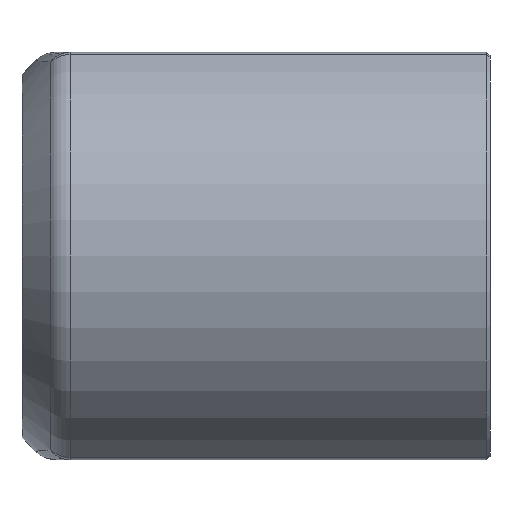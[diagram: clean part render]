
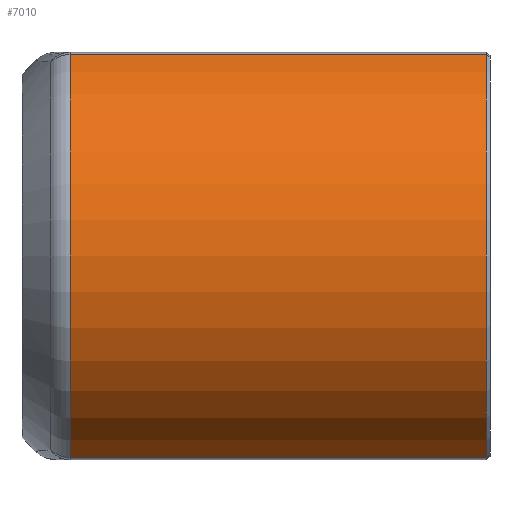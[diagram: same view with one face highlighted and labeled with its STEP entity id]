
A CAD part, front view. The second image highlights one B-rep face of the part: STEP entity #7010.
In plain terms, the highlighted cylindrical face has radius 23.709 mm (diameter 47.418 mm), a partial arc.
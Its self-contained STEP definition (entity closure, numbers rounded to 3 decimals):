
#155 = AXIS2_PLACEMENT_3D ( 'NONE', #1869, #4027, #1839 ) ;
#312 = CARTESIAN_POINT ( 'NONE',  ( -276.425, 16.131, -22.064 ) ) ;
#681 = DIRECTION ( 'NONE',  ( -1., 0., 0. ) ) ;
#938 = VERTEX_POINT ( 'NONE', #7049 ) ;
#957 = FACE_OUTER_BOUND ( 'NONE', #5071, .T. ) ;
#1297 = ORIENTED_EDGE ( 'NONE', *, *, #4584, .F. ) ;
#1752 = VECTOR ( 'NONE', #681, 1000. ) ;
#1839 = DIRECTION ( 'NONE',  ( 0., 0., 1. ) ) ;
#1869 = CARTESIAN_POINT ( 'NONE',  ( -231.416, 25.482, -0.277 ) ) ;
#1878 = LINE ( 'NONE', #5537, #8579 ) ;
#3190 = CARTESIAN_POINT ( 'NONE',  ( -231.416, 16.131, 21.51 ) ) ;
#3499 = CARTESIAN_POINT ( 'NONE',  ( -246.285, 25.482, -0.277 ) ) ;
#3546 = DIRECTION ( 'NONE',  ( -1., 0., 0. ) ) ;
#4027 = DIRECTION ( 'NONE',  ( 1., 0., 0. ) ) ;
#4071 = DIRECTION ( 'NONE',  ( -1., 0., 0. ) ) ;
#4508 = ORIENTED_EDGE ( 'NONE', *, *, #6011, .T. ) ;
#4584 = EDGE_CURVE ( 'NONE', #4763, #6753, #8475, .T. ) ;
#4763 = VERTEX_POINT ( 'NONE', #3190 ) ;
#5071 = EDGE_LOOP ( 'NONE', ( #5627, #5178, #1297, #4508 ) ) ;
#5132 = EDGE_CURVE ( 'NONE', #6753, #5558, #1878, .T. ) ;
#5178 = ORIENTED_EDGE ( 'NONE', *, *, #5132, .F. ) ;
#5341 = CYLINDRICAL_SURFACE ( 'NONE', #7238, 23.709 ) ;
#5537 = CARTESIAN_POINT ( 'NONE',  ( -246.285, 16.131, -22.064 ) ) ;
#5558 = VERTEX_POINT ( 'NONE', #312 ) ;
#5621 = DIRECTION ( 'NONE',  ( 0., 0., 1. ) ) ;
#5627 = ORIENTED_EDGE ( 'NONE', *, *, #8030, .F. ) ;
#6011 = EDGE_CURVE ( 'NONE', #4763, #938, #9044, .T. ) ;
#6753 = VERTEX_POINT ( 'NONE', #8449 ) ;
#6970 = DIRECTION ( 'NONE',  ( -1., 0., 0. ) ) ;
#7010 = ADVANCED_FACE ( 'NONE', ( #957 ), #5341, .T. ) ;
#7049 = CARTESIAN_POINT ( 'NONE',  ( -276.425, 16.131, 21.51 ) ) ;
#7238 = AXIS2_PLACEMENT_3D ( 'NONE', #3499, #6970, #5621 ) ;
#7829 = CARTESIAN_POINT ( 'NONE',  ( -246.285, 16.131, 21.51 ) ) ;
#8030 = EDGE_CURVE ( 'NONE', #5558, #938, #8221, .T. ) ;
#8221 = CIRCLE ( 'NONE', #8323, 23.709 ) ;
#8323 = AXIS2_PLACEMENT_3D ( 'NONE', #8343, #4071, #8433 ) ;
#8343 = CARTESIAN_POINT ( 'NONE',  ( -276.425, 25.482, -0.277 ) ) ;
#8433 = DIRECTION ( 'NONE',  ( 0., -1., 0. ) ) ;
#8449 = CARTESIAN_POINT ( 'NONE',  ( -231.416, 16.131, -22.064 ) ) ;
#8475 = CIRCLE ( 'NONE', #155, 23.709 ) ;
#8579 = VECTOR ( 'NONE', #3546, 1000. ) ;
#9044 = LINE ( 'NONE', #7829, #1752 ) ;
